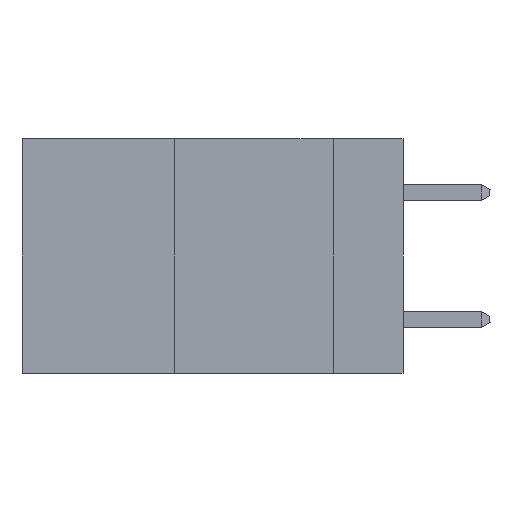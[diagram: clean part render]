
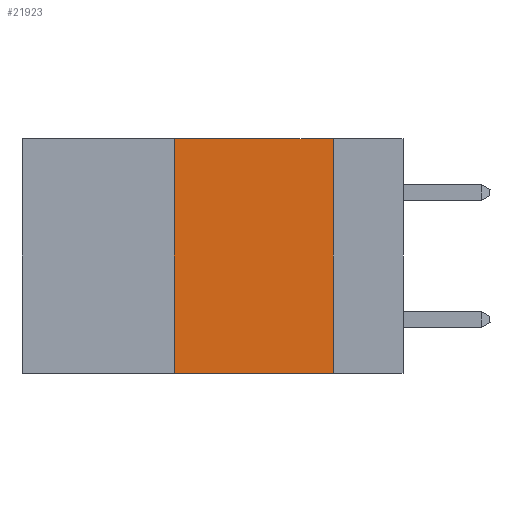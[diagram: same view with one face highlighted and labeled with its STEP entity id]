
A CAD part, left-side view. The second image highlights one B-rep face of the part: STEP entity #21923.
In plain terms, the highlighted planar face has unit normal (-1, 0, 0).
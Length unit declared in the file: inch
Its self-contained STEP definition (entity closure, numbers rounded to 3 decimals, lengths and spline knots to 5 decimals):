
#1177 = CARTESIAN_POINT ( 'NONE',  ( 0., 0.11, -0.37 ) ) ;
#2254 = VERTEX_POINT ( 'NONE', #8558 ) ;
#2266 = ORIENTED_EDGE ( 'NONE', *, *, #37398, .F. ) ;
#4154 = VECTOR ( 'NONE', #22961, 39.37008 ) ;
#7047 = ORIENTED_EDGE ( 'NONE', *, *, #23546, .F. ) ;
#8558 = CARTESIAN_POINT ( 'NONE',  ( 0., 0.36, -0.37 ) ) ;
#8965 = VERTEX_POINT ( 'NONE', #12452 ) ;
#9318 = VECTOR ( 'NONE', #19154, 39.37008 ) ;
#10294 = ORIENTED_EDGE ( 'NONE', *, *, #31304, .F. ) ;
#11698 = LINE ( 'NONE', #16618, #4154 ) ;
#12452 = CARTESIAN_POINT ( 'NONE',  ( 0., 0.36, 0. ) ) ;
#12454 = DIRECTION ( 'NONE',  ( 0., 0., -1. ) ) ;
#12738 = CARTESIAN_POINT ( 'NONE',  ( 0., 0.6, -0.37 ) ) ;
#15066 = PLANE ( 'NONE',  #22260 ) ;
#15702 = EDGE_LOOP ( 'NONE', ( #10294, #7047, #2266, #18552 ) ) ;
#16618 = CARTESIAN_POINT ( 'NONE',  ( 0., 0.36, 0. ) ) ;
#17396 = VECTOR ( 'NONE', #31114, 39.37008 ) ;
#18552 = ORIENTED_EDGE ( 'NONE', *, *, #29897, .T. ) ;
#18929 = CARTESIAN_POINT ( 'NONE',  ( 0., 0.11, 0. ) ) ;
#19010 = CARTESIAN_POINT ( 'NONE',  ( 0., 0.11, 0. ) ) ;
#19025 = CARTESIAN_POINT ( 'NONE',  ( 0., 0.6, 0. ) ) ;
#19154 = DIRECTION ( 'NONE',  ( 0., -1., 0. ) ) ;
#20269 = LINE ( 'NONE', #19025, #17396 ) ;
#21462 = DIRECTION ( 'NONE',  ( 0., 0., -1. ) ) ;
#21775 = FACE_OUTER_BOUND ( 'NONE', #15702, .T. ) ;
#21923 = ADVANCED_FACE ( 'NONE', ( #21775 ), #15066, .F. ) ;
#22260 = AXIS2_PLACEMENT_3D ( 'NONE', #30468, #36363, #12454 ) ;
#22961 = DIRECTION ( 'NONE',  ( 0., 0., 1. ) ) ;
#23546 = EDGE_CURVE ( 'NONE', #8965, #31938, #20269, .T. ) ;
#25678 = LINE ( 'NONE', #18929, #30374 ) ;
#29117 = LINE ( 'NONE', #12738, #9318 ) ;
#29897 = EDGE_CURVE ( 'NONE', #2254, #34243, #29117, .T. ) ;
#30374 = VECTOR ( 'NONE', #21462, 39.37008 ) ;
#30468 = CARTESIAN_POINT ( 'NONE',  ( 0., 0.6, 0. ) ) ;
#31114 = DIRECTION ( 'NONE',  ( 0., -1., 0. ) ) ;
#31304 = EDGE_CURVE ( 'NONE', #31938, #34243, #25678, .T. ) ;
#31938 = VERTEX_POINT ( 'NONE', #19010 ) ;
#34243 = VERTEX_POINT ( 'NONE', #1177 ) ;
#36363 = DIRECTION ( 'NONE',  ( 1., 0., 0. ) ) ;
#37398 = EDGE_CURVE ( 'NONE', #2254, #8965, #11698, .T. ) ;
